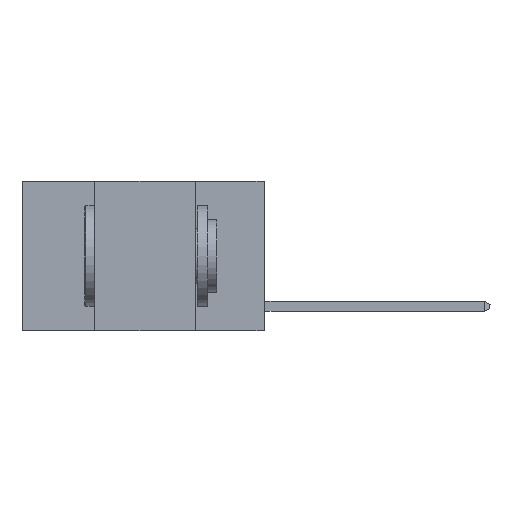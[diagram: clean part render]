
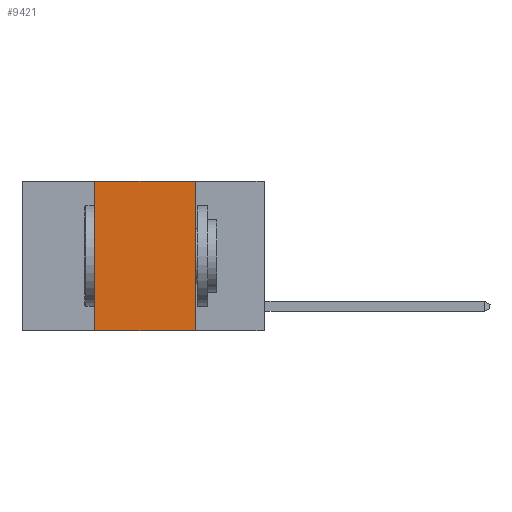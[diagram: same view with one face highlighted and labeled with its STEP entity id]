
A CAD part, left-side view. The second image highlights one B-rep face of the part: STEP entity #9421.
In plain terms, the highlighted planar face has unit normal (-1, 0, 0).
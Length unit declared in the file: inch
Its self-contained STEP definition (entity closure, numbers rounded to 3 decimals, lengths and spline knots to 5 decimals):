
#466 = DIRECTION ( 'NONE',  ( 0., 0., 1. ) ) ;
#653 = DIRECTION ( 'NONE',  ( 1., 0., 0. ) ) ;
#689 = EDGE_CURVE ( 'NONE', #5716, #12350, #9043, .T. ) ;
#730 = DIRECTION ( 'NONE',  ( 0., 0., -1. ) ) ;
#1012 = VERTEX_POINT ( 'NONE', #1357 ) ;
#1198 = VECTOR ( 'NONE', #13163, 39.37008 ) ;
#1357 = CARTESIAN_POINT ( 'NONE',  ( 0., 0.42, 0. ) ) ;
#1685 = CARTESIAN_POINT ( 'NONE',  ( 0., 0.6, 0. ) ) ;
#2482 = EDGE_LOOP ( 'NONE', ( #12946, #6016, #9561, #3518 ) ) ;
#3518 = ORIENTED_EDGE ( 'NONE', *, *, #689, .T. ) ;
#3849 = CARTESIAN_POINT ( 'NONE',  ( 0., 0.6, 0. ) ) ;
#4550 = DIRECTION ( 'NONE',  ( 0., -1., 0. ) ) ;
#5111 = LINE ( 'NONE', #3849, #1198 ) ;
#5161 = VECTOR ( 'NONE', #466, 39.37008 ) ;
#5716 = VERTEX_POINT ( 'NONE', #9951 ) ;
#6016 = ORIENTED_EDGE ( 'NONE', *, *, #13705, .F. ) ;
#7244 = LINE ( 'NONE', #8585, #13587 ) ;
#7614 = CARTESIAN_POINT ( 'NONE',  ( 0., 0.17, -0.37 ) ) ;
#7668 = CARTESIAN_POINT ( 'NONE',  ( 0., 0.42, 0. ) ) ;
#7698 = AXIS2_PLACEMENT_3D ( 'NONE', #1685, #653, #730 ) ;
#8465 = VECTOR ( 'NONE', #4550, 39.37008 ) ;
#8585 = CARTESIAN_POINT ( 'NONE',  ( 0., 0.17, 0. ) ) ;
#8655 = EDGE_CURVE ( 'NONE', #5716, #1012, #14863, .T. ) ;
#9043 = LINE ( 'NONE', #15130, #8465 ) ;
#9421 = ADVANCED_FACE ( 'NONE', ( #11560 ), #11481, .F. ) ;
#9561 = ORIENTED_EDGE ( 'NONE', *, *, #8655, .F. ) ;
#9951 = CARTESIAN_POINT ( 'NONE',  ( 0., 0.42, -0.37 ) ) ;
#11481 = PLANE ( 'NONE',  #7698 ) ;
#11560 = FACE_OUTER_BOUND ( 'NONE', #2482, .T. ) ;
#12350 = VERTEX_POINT ( 'NONE', #7614 ) ;
#12946 = ORIENTED_EDGE ( 'NONE', *, *, #15078, .F. ) ;
#13163 = DIRECTION ( 'NONE',  ( 0., -1., 0. ) ) ;
#13394 = DIRECTION ( 'NONE',  ( 0., 0., -1. ) ) ;
#13587 = VECTOR ( 'NONE', #13394, 39.37008 ) ;
#13705 = EDGE_CURVE ( 'NONE', #1012, #14088, #5111, .T. ) ;
#14088 = VERTEX_POINT ( 'NONE', #14857 ) ;
#14857 = CARTESIAN_POINT ( 'NONE',  ( 0., 0.17, 0. ) ) ;
#14863 = LINE ( 'NONE', #7668, #5161 ) ;
#15078 = EDGE_CURVE ( 'NONE', #14088, #12350, #7244, .T. ) ;
#15130 = CARTESIAN_POINT ( 'NONE',  ( 0., 0.6, -0.37 ) ) ;
